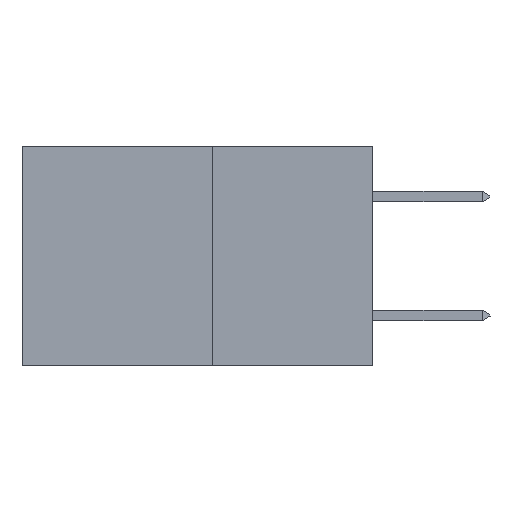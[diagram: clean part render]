
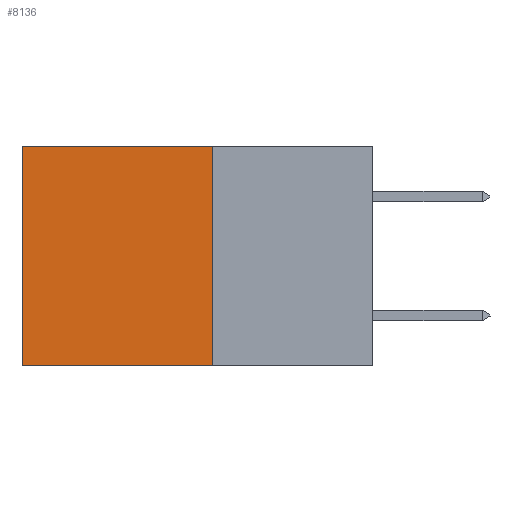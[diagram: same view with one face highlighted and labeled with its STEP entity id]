
A CAD part, left-side view. The second image highlights one B-rep face of the part: STEP entity #8136.
In plain terms, the highlighted planar face has unit normal (-1, 0, 0).
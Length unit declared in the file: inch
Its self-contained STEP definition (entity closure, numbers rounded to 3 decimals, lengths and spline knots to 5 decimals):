
#149 = VECTOR ( 'NONE', #5953, 39.37008 ) ;
#289 = ORIENTED_EDGE ( 'NONE', *, *, #642, .F. ) ;
#484 = ORIENTED_EDGE ( 'NONE', *, *, #10492, .T. ) ;
#517 = FACE_OUTER_BOUND ( 'NONE', #7603, .T. ) ;
#620 = DIRECTION ( 'NONE',  ( 0., 0., -1. ) ) ;
#642 = EDGE_CURVE ( 'NONE', #9725, #11018, #6893, .T. ) ;
#1879 = VECTOR ( 'NONE', #620, 39.37008 ) ;
#2518 = AXIS2_PLACEMENT_3D ( 'NONE', #4986, #11133, #5131 ) ;
#2696 = CARTESIAN_POINT ( 'NONE',  ( 0.277, 0.27, 0. ) ) ;
#2750 = LINE ( 'NONE', #2820, #7445 ) ;
#2820 = CARTESIAN_POINT ( 'NONE',  ( 0.277, 0.27, -0.37 ) ) ;
#3634 = VERTEX_POINT ( 'NONE', #10988 ) ;
#4151 = DIRECTION ( 'NONE',  ( 0., 1., 0. ) ) ;
#4936 = CARTESIAN_POINT ( 'NONE',  ( 0.277, 0.59, -0.37 ) ) ;
#4986 = CARTESIAN_POINT ( 'NONE',  ( 0.277, 0.27, -0.37 ) ) ;
#5053 = CARTESIAN_POINT ( 'NONE',  ( 0.277, 0.27, 0. ) ) ;
#5131 = DIRECTION ( 'NONE',  ( 0., 0., -1. ) ) ;
#5552 = DIRECTION ( 'NONE',  ( 0., 0., -1. ) ) ;
#5906 = ORIENTED_EDGE ( 'NONE', *, *, #7028, .F. ) ;
#5953 = DIRECTION ( 'NONE',  ( 0., 1., 0. ) ) ;
#5967 = EDGE_CURVE ( 'NONE', #3634, #8315, #9486, .T. ) ;
#6625 = PLANE ( 'NONE',  #2518 ) ;
#6893 = LINE ( 'NONE', #9209, #1879 ) ;
#7028 = EDGE_CURVE ( 'NONE', #11018, #8315, #2750, .T. ) ;
#7445 = VECTOR ( 'NONE', #4151, 39.37008 ) ;
#7603 = EDGE_LOOP ( 'NONE', ( #11722, #5906, #289, #484 ) ) ;
#7742 = CARTESIAN_POINT ( 'NONE',  ( 0.277, 0.27, -0.37 ) ) ;
#7802 = LINE ( 'NONE', #5053, #149 ) ;
#8136 = ADVANCED_FACE ( 'NONE', ( #517 ), #6625, .F. ) ;
#8315 = VERTEX_POINT ( 'NONE', #9117 ) ;
#8908 = VECTOR ( 'NONE', #5552, 39.37008 ) ;
#9117 = CARTESIAN_POINT ( 'NONE',  ( 0.277, 0.59, -0.37 ) ) ;
#9209 = CARTESIAN_POINT ( 'NONE',  ( 0.277, 0.27, -0.37 ) ) ;
#9486 = LINE ( 'NONE', #4936, #8908 ) ;
#9725 = VERTEX_POINT ( 'NONE', #2696 ) ;
#10492 = EDGE_CURVE ( 'NONE', #9725, #3634, #7802, .T. ) ;
#10988 = CARTESIAN_POINT ( 'NONE',  ( 0.277, 0.59, 0. ) ) ;
#11018 = VERTEX_POINT ( 'NONE', #7742 ) ;
#11133 = DIRECTION ( 'NONE',  ( 1., 0., 0. ) ) ;
#11722 = ORIENTED_EDGE ( 'NONE', *, *, #5967, .T. ) ;
